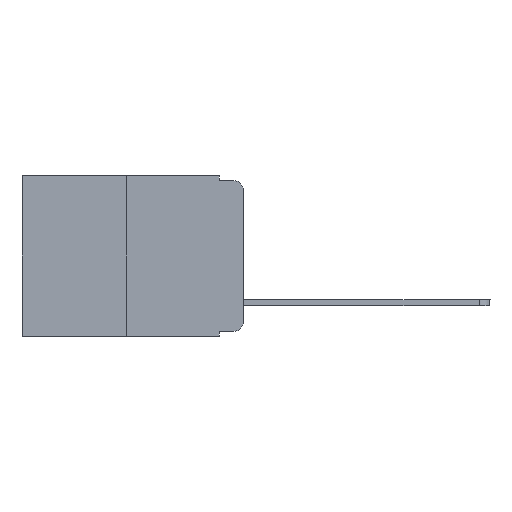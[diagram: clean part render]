
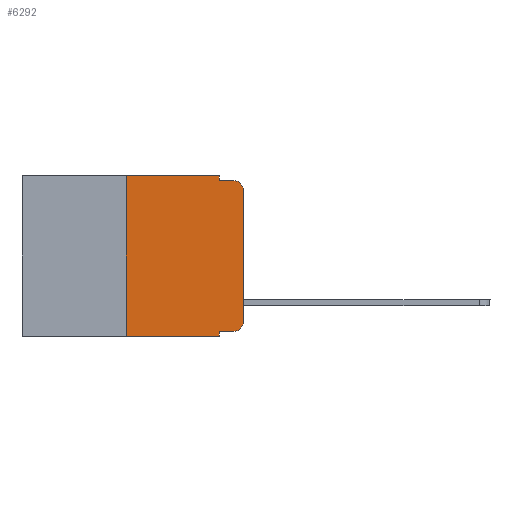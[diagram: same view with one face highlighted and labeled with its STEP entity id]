
A CAD part, left-side view. The second image highlights one B-rep face of the part: STEP entity #6292.
In plain terms, the highlighted planar face has unit normal (-1, 0, 0).
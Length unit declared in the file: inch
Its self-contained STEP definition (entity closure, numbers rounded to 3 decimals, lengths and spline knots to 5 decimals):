
#515 = CARTESIAN_POINT ( 'NONE',  ( 0., 0.051, -0.333 ) ) ;
#583 = AXIS2_PLACEMENT_3D ( 'NONE', #11775, #13696, #15359 ) ;
#1203 = VERTEX_POINT ( 'NONE', #515 ) ;
#1274 = EDGE_CURVE ( 'NONE', #7094, #2151, #19548, .T. ) ;
#1420 = DIRECTION ( 'NONE',  ( 0., -1., 0. ) ) ;
#1423 = EDGE_CURVE ( 'NONE', #8744, #17499, #23673, .T. ) ;
#1462 = VERTEX_POINT ( 'NONE', #7042 ) ;
#1892 = ORIENTED_EDGE ( 'NONE', *, *, #8698, .T. ) ;
#2151 = VERTEX_POINT ( 'NONE', #13261 ) ;
#2430 = CARTESIAN_POINT ( 'NONE',  ( 0., 0.25, -0.343 ) ) ;
#2504 = ORIENTED_EDGE ( 'NONE', *, *, #22787, .T. ) ;
#2615 = DIRECTION ( 'NONE',  ( 0., 0., 1. ) ) ;
#3056 = LINE ( 'NONE', #16744, #22678 ) ;
#3361 = VERTEX_POINT ( 'NONE', #21066 ) ;
#3567 = FACE_OUTER_BOUND ( 'NONE', #24050, .T. ) ;
#3848 = DIRECTION ( 'NONE',  ( -1., 0., 0. ) ) ;
#3981 = VECTOR ( 'NONE', #10592, 39.37008 ) ;
#4433 = LINE ( 'NONE', #20964, #18467 ) ;
#4612 = CARTESIAN_POINT ( 'NONE',  ( 0., 0., 0. ) ) ;
#5811 = DIRECTION ( 'NONE',  ( 0., -1., 0. ) ) ;
#5859 = DIRECTION ( 'NONE',  ( -1., 0., 0. ) ) ;
#6292 = ADVANCED_FACE ( 'NONE', ( #3567 ), #11688, .F. ) ;
#6634 = CARTESIAN_POINT ( 'NONE',  ( 0., 0.02, -0.333 ) ) ;
#7042 = CARTESIAN_POINT ( 'NONE',  ( 0., 0.051, -0.343 ) ) ;
#7094 = VERTEX_POINT ( 'NONE', #2430 ) ;
#7262 = AXIS2_PLACEMENT_3D ( 'NONE', #18626, #5859, #21089 ) ;
#7315 = CARTESIAN_POINT ( 'NONE',  ( 0., 0.051, -0.01 ) ) ;
#7607 = DIRECTION ( 'NONE',  ( 0., 0., -1. ) ) ;
#8665 = ORIENTED_EDGE ( 'NONE', *, *, #11944, .T. ) ;
#8698 = EDGE_CURVE ( 'NONE', #7094, #1462, #9713, .T. ) ;
#8744 = VERTEX_POINT ( 'NONE', #16683 ) ;
#8794 = DIRECTION ( 'NONE',  ( 0., -1., 0. ) ) ;
#9240 = EDGE_CURVE ( 'NONE', #1203, #17918, #23607, .T. ) ;
#9713 = LINE ( 'NONE', #16434, #20445 ) ;
#10592 = DIRECTION ( 'NONE',  ( 0., -1., 0. ) ) ;
#11688 = PLANE ( 'NONE',  #583 ) ;
#11775 = CARTESIAN_POINT ( 'NONE',  ( 0., 0.473, 0. ) ) ;
#11944 = EDGE_CURVE ( 'NONE', #17918, #15086, #17890, .T. ) ;
#11957 = CARTESIAN_POINT ( 'NONE',  ( 0., 0.25, 0. ) ) ;
#12781 = DIRECTION ( 'NONE',  ( 0., 0., -1. ) ) ;
#12976 = VERTEX_POINT ( 'NONE', #21657 ) ;
#13080 = ORIENTED_EDGE ( 'NONE', *, *, #14271, .T. ) ;
#13122 = VECTOR ( 'NONE', #1420, 39.37008 ) ;
#13261 = CARTESIAN_POINT ( 'NONE',  ( 0., 0.25, 0. ) ) ;
#13269 = VECTOR ( 'NONE', #17942, 39.37008 ) ;
#13450 = ORIENTED_EDGE ( 'NONE', *, *, #9240, .T. ) ;
#13554 = CARTESIAN_POINT ( 'NONE',  ( 0., 0., -0.313 ) ) ;
#13589 = VECTOR ( 'NONE', #12781, 39.37008 ) ;
#13696 = DIRECTION ( 'NONE',  ( 1., 0., 0. ) ) ;
#13703 = ORIENTED_EDGE ( 'NONE', *, *, #21560, .F. ) ;
#14016 = LINE ( 'NONE', #16607, #13122 ) ;
#14271 = EDGE_CURVE ( 'NONE', #15086, #12976, #21250, .T. ) ;
#14486 = ORIENTED_EDGE ( 'NONE', *, *, #1423, .F. ) ;
#14917 = DIRECTION ( 'NONE',  ( 0., 0., -1. ) ) ;
#15003 = VECTOR ( 'NONE', #2615, 39.37008 ) ;
#15086 = VERTEX_POINT ( 'NONE', #13554 ) ;
#15359 = DIRECTION ( 'NONE',  ( 0., 0., -1. ) ) ;
#16108 = ORIENTED_EDGE ( 'NONE', *, *, #24008, .F. ) ;
#16293 = EDGE_CURVE ( 'NONE', #17499, #3361, #14016, .T. ) ;
#16434 = CARTESIAN_POINT ( 'NONE',  ( 0., 0.473, -0.343 ) ) ;
#16607 = CARTESIAN_POINT ( 'NONE',  ( 0., 0.051, -0.01 ) ) ;
#16683 = CARTESIAN_POINT ( 'NONE',  ( 0., 0.051, 0. ) ) ;
#16744 = CARTESIAN_POINT ( 'NONE',  ( 0., 0.051, 0. ) ) ;
#17097 = CARTESIAN_POINT ( 'NONE',  ( 0., 0.02, -0.313 ) ) ;
#17308 = CIRCLE ( 'NONE', #7262, 0.02 ) ;
#17499 = VERTEX_POINT ( 'NONE', #7315 ) ;
#17890 = CIRCLE ( 'NONE', #17962, 0.02 ) ;
#17918 = VERTEX_POINT ( 'NONE', #6634 ) ;
#17942 = DIRECTION ( 'NONE',  ( 0., 0., 1. ) ) ;
#17962 = AXIS2_PLACEMENT_3D ( 'NONE', #17097, #3848, #7607 ) ;
#18467 = VECTOR ( 'NONE', #5811, 39.37008 ) ;
#18626 = CARTESIAN_POINT ( 'NONE',  ( 0., 0.02, -0.03 ) ) ;
#19548 = LINE ( 'NONE', #11957, #13269 ) ;
#20445 = VECTOR ( 'NONE', #8794, 39.37008 ) ;
#20964 = CARTESIAN_POINT ( 'NONE',  ( 0., 0.473, 0. ) ) ;
#21030 = ORIENTED_EDGE ( 'NONE', *, *, #1274, .F. ) ;
#21066 = CARTESIAN_POINT ( 'NONE',  ( 0., 0.02, -0.01 ) ) ;
#21089 = DIRECTION ( 'NONE',  ( 0., 0., -1. ) ) ;
#21250 = LINE ( 'NONE', #4612, #15003 ) ;
#21560 = EDGE_CURVE ( 'NONE', #1203, #1462, #3056, .T. ) ;
#21657 = CARTESIAN_POINT ( 'NONE',  ( 0., 0., -0.03 ) ) ;
#21967 = CARTESIAN_POINT ( 'NONE',  ( 0., 0.051, -0.333 ) ) ;
#22258 = CARTESIAN_POINT ( 'NONE',  ( 0., 0.051, 0. ) ) ;
#22678 = VECTOR ( 'NONE', #14917, 39.37008 ) ;
#22787 = EDGE_CURVE ( 'NONE', #12976, #3361, #17308, .T. ) ;
#23147 = ORIENTED_EDGE ( 'NONE', *, *, #16293, .F. ) ;
#23607 = LINE ( 'NONE', #21967, #3981 ) ;
#23673 = LINE ( 'NONE', #22258, #13589 ) ;
#24008 = EDGE_CURVE ( 'NONE', #2151, #8744, #4433, .T. ) ;
#24050 = EDGE_LOOP ( 'NONE', ( #13080, #2504, #23147, #14486, #16108, #21030, #1892, #13703, #13450, #8665 ) ) ;
